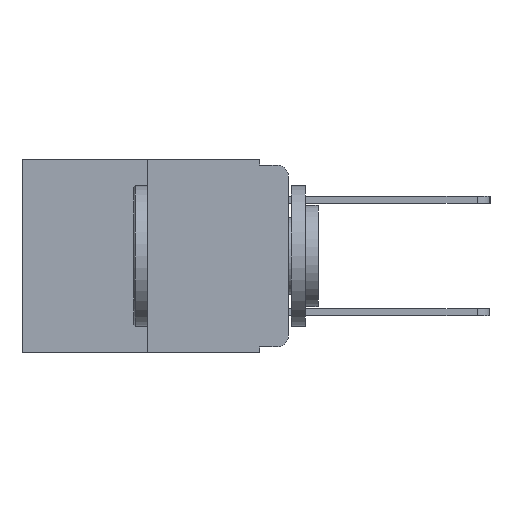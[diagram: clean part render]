
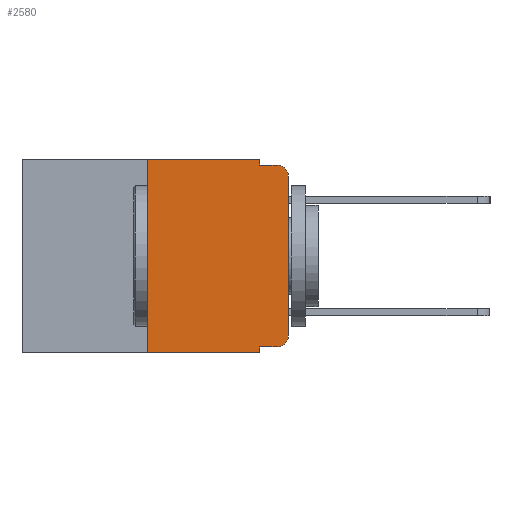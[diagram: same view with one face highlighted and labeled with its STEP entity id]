
A CAD part, left-side view. The second image highlights one B-rep face of the part: STEP entity #2580.
In plain terms, the highlighted planar face has unit normal (-1, 0, 0).
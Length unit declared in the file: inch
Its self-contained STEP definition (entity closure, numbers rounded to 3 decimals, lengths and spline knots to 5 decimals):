
#276 = DIRECTION ( 'NONE',  ( 0., -1., 0. ) ) ;
#305 = VERTEX_POINT ( 'NONE', #8355 ) ;
#753 = VECTOR ( 'NONE', #276, 39.37008 ) ;
#762 = CARTESIAN_POINT ( 'NONE',  ( 0., 0.051, -0.333 ) ) ;
#938 = VERTEX_POINT ( 'NONE', #14760 ) ;
#1205 = CIRCLE ( 'NONE', #9737, 0.02 ) ;
#1592 = CARTESIAN_POINT ( 'NONE',  ( 0., 0.02, -0.01 ) ) ;
#1607 = CARTESIAN_POINT ( 'NONE',  ( 0., 0.02, -0.333 ) ) ;
#1714 = LINE ( 'NONE', #11622, #10760 ) ;
#1923 = LINE ( 'NONE', #4428, #5300 ) ;
#2360 = VERTEX_POINT ( 'NONE', #5685 ) ;
#2457 = VECTOR ( 'NONE', #9635, 39.37008 ) ;
#2580 = ADVANCED_FACE ( 'NONE', ( #2810 ), #4127, .F. ) ;
#2611 = EDGE_CURVE ( 'NONE', #12129, #2757, #1923, .T. ) ;
#2627 = CARTESIAN_POINT ( 'NONE',  ( 0., 0.473, 0. ) ) ;
#2757 = VERTEX_POINT ( 'NONE', #1607 ) ;
#2759 = VERTEX_POINT ( 'NONE', #1592 ) ;
#2810 = FACE_OUTER_BOUND ( 'NONE', #8580, .T. ) ;
#3181 = CARTESIAN_POINT ( 'NONE',  ( 0., 0., -0.03 ) ) ;
#3733 = DIRECTION ( 'NONE',  ( 0., 0., -1. ) ) ;
#3770 = CARTESIAN_POINT ( 'NONE',  ( 0., 0.02, -0.03 ) ) ;
#4030 = DIRECTION ( 'NONE',  ( 0., 0., -1. ) ) ;
#4038 = DIRECTION ( 'NONE',  ( 1., 0., 0. ) ) ;
#4127 = PLANE ( 'NONE',  #11972 ) ;
#4262 = DIRECTION ( 'NONE',  ( 0., 0., -1. ) ) ;
#4409 = DIRECTION ( 'NONE',  ( 0., -1., 0. ) ) ;
#4428 = CARTESIAN_POINT ( 'NONE',  ( 0., 0.051, -0.333 ) ) ;
#4476 = ORIENTED_EDGE ( 'NONE', *, *, #5711, .T. ) ;
#4506 = CARTESIAN_POINT ( 'NONE',  ( 0., 0.02, -0.313 ) ) ;
#4698 = CARTESIAN_POINT ( 'NONE',  ( 0., 0.051, -0.01 ) ) ;
#4782 = VERTEX_POINT ( 'NONE', #12671 ) ;
#4807 = VECTOR ( 'NONE', #14232, 39.37008 ) ;
#4847 = VERTEX_POINT ( 'NONE', #3181 ) ;
#5300 = VECTOR ( 'NONE', #4409, 39.37008 ) ;
#5655 = DIRECTION ( 'NONE',  ( 0., 0., -1. ) ) ;
#5685 = CARTESIAN_POINT ( 'NONE',  ( 0., 0., -0.313 ) ) ;
#5711 = EDGE_CURVE ( 'NONE', #12467, #4782, #10396, .T. ) ;
#5729 = ORIENTED_EDGE ( 'NONE', *, *, #12139, .T. ) ;
#6088 = ORIENTED_EDGE ( 'NONE', *, *, #10298, .T. ) ;
#6268 = CARTESIAN_POINT ( 'NONE',  ( 0., 0.25, -0.343 ) ) ;
#6462 = LINE ( 'NONE', #14349, #8801 ) ;
#6631 = CIRCLE ( 'NONE', #7656, 0.02 ) ;
#7309 = EDGE_CURVE ( 'NONE', #12467, #9650, #8062, .T. ) ;
#7403 = EDGE_CURVE ( 'NONE', #2757, #2360, #6631, .T. ) ;
#7656 = AXIS2_PLACEMENT_3D ( 'NONE', #4506, #12254, #5655 ) ;
#7757 = EDGE_CURVE ( 'NONE', #9650, #938, #12257, .T. ) ;
#8062 = LINE ( 'NONE', #10006, #10644 ) ;
#8076 = EDGE_CURVE ( 'NONE', #12129, #4782, #13514, .T. ) ;
#8266 = ORIENTED_EDGE ( 'NONE', *, *, #2611, .T. ) ;
#8355 = CARTESIAN_POINT ( 'NONE',  ( 0., 0.051, -0.01 ) ) ;
#8580 = EDGE_LOOP ( 'NONE', ( #5729, #6088, #9146, #11960, #12615, #12937, #4476, #10835, #8266, #13882 ) ) ;
#8801 = VECTOR ( 'NONE', #10264, 39.37008 ) ;
#9052 = CARTESIAN_POINT ( 'NONE',  ( 0., 0.051, 0. ) ) ;
#9146 = ORIENTED_EDGE ( 'NONE', *, *, #14865, .F. ) ;
#9583 = EDGE_CURVE ( 'NONE', #938, #305, #1714, .T. ) ;
#9635 = DIRECTION ( 'NONE',  ( 0., -1., 0. ) ) ;
#9650 = VERTEX_POINT ( 'NONE', #14789 ) ;
#9737 = AXIS2_PLACEMENT_3D ( 'NONE', #3770, #11018, #4262 ) ;
#10006 = CARTESIAN_POINT ( 'NONE',  ( 0., 0.25, 0. ) ) ;
#10264 = DIRECTION ( 'NONE',  ( 0., 0., 1. ) ) ;
#10298 = EDGE_CURVE ( 'NONE', #4847, #2759, #1205, .T. ) ;
#10396 = LINE ( 'NONE', #14175, #753 ) ;
#10644 = VECTOR ( 'NONE', #13108, 39.37008 ) ;
#10760 = VECTOR ( 'NONE', #3733, 39.37008 ) ;
#10835 = ORIENTED_EDGE ( 'NONE', *, *, #8076, .F. ) ;
#11018 = DIRECTION ( 'NONE',  ( -1., 0., 0. ) ) ;
#11622 = CARTESIAN_POINT ( 'NONE',  ( 0., 0.051, 0. ) ) ;
#11960 = ORIENTED_EDGE ( 'NONE', *, *, #9583, .F. ) ;
#11966 = CARTESIAN_POINT ( 'NONE',  ( 0., 0.473, 0. ) ) ;
#11972 = AXIS2_PLACEMENT_3D ( 'NONE', #11966, #4038, #4030 ) ;
#12129 = VERTEX_POINT ( 'NONE', #762 ) ;
#12139 = EDGE_CURVE ( 'NONE', #2360, #4847, #6462, .T. ) ;
#12254 = DIRECTION ( 'NONE',  ( -1., 0., 0. ) ) ;
#12257 = LINE ( 'NONE', #2627, #2457 ) ;
#12467 = VERTEX_POINT ( 'NONE', #6268 ) ;
#12615 = ORIENTED_EDGE ( 'NONE', *, *, #7757, .F. ) ;
#12671 = CARTESIAN_POINT ( 'NONE',  ( 0., 0.051, -0.343 ) ) ;
#12937 = ORIENTED_EDGE ( 'NONE', *, *, #7309, .F. ) ;
#13108 = DIRECTION ( 'NONE',  ( 0., 0., 1. ) ) ;
#13432 = VECTOR ( 'NONE', #14409, 39.37008 ) ;
#13514 = LINE ( 'NONE', #9052, #4807 ) ;
#13759 = LINE ( 'NONE', #4698, #13432 ) ;
#13882 = ORIENTED_EDGE ( 'NONE', *, *, #7403, .T. ) ;
#14175 = CARTESIAN_POINT ( 'NONE',  ( 0., 0.473, -0.343 ) ) ;
#14232 = DIRECTION ( 'NONE',  ( 0., 0., -1. ) ) ;
#14349 = CARTESIAN_POINT ( 'NONE',  ( 0., 0., 0. ) ) ;
#14409 = DIRECTION ( 'NONE',  ( 0., -1., 0. ) ) ;
#14760 = CARTESIAN_POINT ( 'NONE',  ( 0., 0.051, 0. ) ) ;
#14789 = CARTESIAN_POINT ( 'NONE',  ( 0., 0.25, 0. ) ) ;
#14865 = EDGE_CURVE ( 'NONE', #305, #2759, #13759, .T. ) ;
